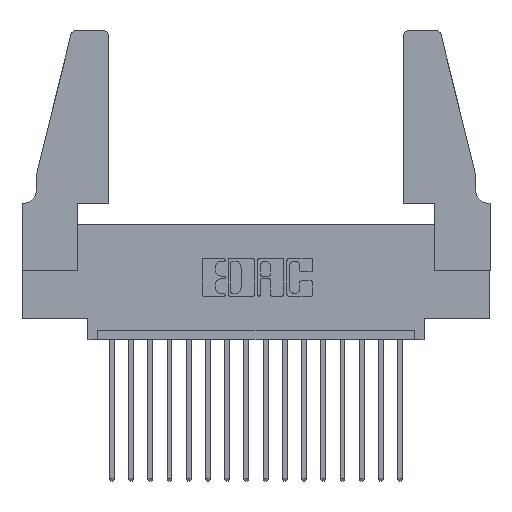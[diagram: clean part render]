
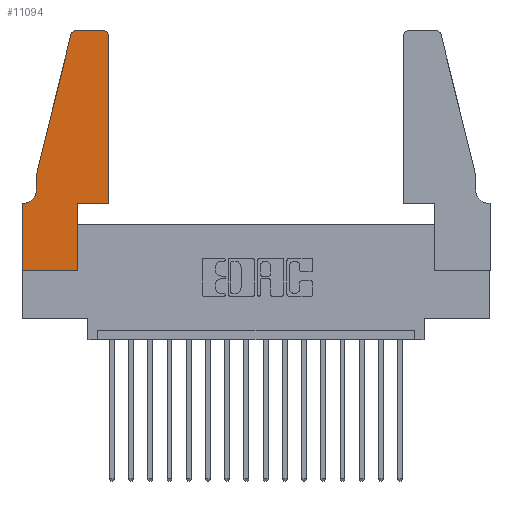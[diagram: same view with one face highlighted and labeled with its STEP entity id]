
A CAD part, top view. The second image highlights one B-rep face of the part: STEP entity #11094.
In plain terms, the highlighted planar face has unit normal (0, 0, 1).
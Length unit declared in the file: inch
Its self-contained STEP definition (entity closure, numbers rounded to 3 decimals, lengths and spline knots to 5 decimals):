
#214 = CARTESIAN_POINT ( 'NONE',  ( 0., 0., 0.37 ) ) ;
#516 = CARTESIAN_POINT ( 'NONE',  ( 0.4505, 0.35, 0.37 ) ) ;
#1029 = VECTOR ( 'NONE', #11765, 39.37008 ) ;
#1052 = EDGE_CURVE ( 'NONE', #11548, #11815, #8844, .T. ) ;
#1663 = VERTEX_POINT ( 'NONE', #3851 ) ;
#1678 = CARTESIAN_POINT ( 'NONE',  ( 0.2865, 0., 0.37 ) ) ;
#1750 = LINE ( 'NONE', #7636, #5211 ) ;
#2048 = LINE ( 'NONE', #2985, #11067 ) ;
#2205 = DIRECTION ( 'NONE',  ( 1., 0., 0. ) ) ;
#2269 = EDGE_LOOP ( 'NONE', ( #16518, #8946, #4873, #13124, #3448, #4816, #2460, #8120, #2951, #8893, #3807, #16156 ) ) ;
#2369 = DIRECTION ( 'NONE',  ( 0., 0., 1. ) ) ;
#2460 = ORIENTED_EDGE ( 'NONE', *, *, #16894, .T. ) ;
#2951 = ORIENTED_EDGE ( 'NONE', *, *, #15072, .T. ) ;
#2985 = CARTESIAN_POINT ( 'NONE',  ( 0.0755, 0.35, 0.37 ) ) ;
#3305 = VERTEX_POINT ( 'NONE', #4848 ) ;
#3448 = ORIENTED_EDGE ( 'NONE', *, *, #11821, .T. ) ;
#3489 = DIRECTION ( 'NONE',  ( 0., 1., 0. ) ) ;
#3698 = CARTESIAN_POINT ( 'NONE',  ( 0., 0.35, 0.37 ) ) ;
#3749 = VECTOR ( 'NONE', #5979, 39.37008 ) ;
#3807 = ORIENTED_EDGE ( 'NONE', *, *, #10833, .T. ) ;
#3851 = CARTESIAN_POINT ( 'NONE',  ( 0.284, 1.25, 0.37 ) ) ;
#4816 = ORIENTED_EDGE ( 'NONE', *, *, #7312, .T. ) ;
#4840 = CARTESIAN_POINT ( 'NONE',  ( 0., 0., 0.37 ) ) ;
#4848 = CARTESIAN_POINT ( 'NONE',  ( 0.0055, 0.35, 0.37 ) ) ;
#4873 = ORIENTED_EDGE ( 'NONE', *, *, #17063, .T. ) ;
#4964 = VERTEX_POINT ( 'NONE', #4840 ) ;
#4983 = EDGE_CURVE ( 'NONE', #17170, #1663, #16976, .T. ) ;
#5161 = DIRECTION ( 'NONE',  ( 1., 0., 0. ) ) ;
#5211 = VECTOR ( 'NONE', #3489, 39.37008 ) ;
#5729 = AXIS2_PLACEMENT_3D ( 'NONE', #15974, #15744, #11642 ) ;
#5944 = CARTESIAN_POINT ( 'NONE',  ( 0.2865, 0.35, 0.37 ) ) ;
#5979 = DIRECTION ( 'NONE',  ( 0., -1., 0. ) ) ;
#6034 = CARTESIAN_POINT ( 'NONE',  ( 0.4505, 0.35, 0.37 ) ) ;
#6447 = CARTESIAN_POINT ( 'NONE',  ( 0.0055, 0.42, 0.37 ) ) ;
#6463 = DIRECTION ( 'NONE',  ( -1., 0., 0. ) ) ;
#6544 = DIRECTION ( 'NONE',  ( 1., 0., 0. ) ) ;
#6773 = LINE ( 'NONE', #214, #3749 ) ;
#6805 = AXIS2_PLACEMENT_3D ( 'NONE', #12124, #14798, #6544 ) ;
#7031 = CIRCLE ( 'NONE', #11001, 0.07 ) ;
#7102 = CARTESIAN_POINT ( 'NONE',  ( 0., 0.35, 0.37 ) ) ;
#7312 = EDGE_CURVE ( 'NONE', #3305, #14896, #2048, .T. ) ;
#7475 = VECTOR ( 'NONE', #2205, 39.37008 ) ;
#7476 = VERTEX_POINT ( 'NONE', #6034 ) ;
#7528 = CARTESIAN_POINT ( 'NONE',  ( 0.0755, 0.5, 0.37 ) ) ;
#7577 = CARTESIAN_POINT ( 'NONE',  ( 0.0755, 0.5, 0.37 ) ) ;
#7585 = CARTESIAN_POINT ( 'NONE',  ( 0.2605, 1.25, 0.37 ) ) ;
#7636 = CARTESIAN_POINT ( 'NONE',  ( 0.2865, 0.35, 0.37 ) ) ;
#7899 = VECTOR ( 'NONE', #17232, 39.37008 ) ;
#8120 = ORIENTED_EDGE ( 'NONE', *, *, #15819, .T. ) ;
#8230 = AXIS2_PLACEMENT_3D ( 'NONE', #3698, #2369, #5161 ) ;
#8292 = CIRCLE ( 'NONE', #6805, 0.03 ) ;
#8754 = LINE ( 'NONE', #9001, #7475 ) ;
#8817 = DIRECTION ( 'NONE',  ( 1., 0., 0. ) ) ;
#8844 = LINE ( 'NONE', #7528, #13807 ) ;
#8893 = ORIENTED_EDGE ( 'NONE', *, *, #17524, .T. ) ;
#8946 = ORIENTED_EDGE ( 'NONE', *, *, #11992, .T. ) ;
#9001 = CARTESIAN_POINT ( 'NONE',  ( 0., 0., 0.37 ) ) ;
#9907 = VERTEX_POINT ( 'NONE', #5944 ) ;
#10202 = VECTOR ( 'NONE', #8817, 39.37008 ) ;
#10833 = EDGE_CURVE ( 'NONE', #7476, #11523, #12900, .T. ) ;
#11001 = AXIS2_PLACEMENT_3D ( 'NONE', #6447, #14585, #13121 ) ;
#11067 = VECTOR ( 'NONE', #6463, 39.37008 ) ;
#11094 = ADVANCED_FACE ( 'NONE', ( #14184 ), #13445, .T. ) ;
#11523 = VERTEX_POINT ( 'NONE', #12612 ) ;
#11548 = VERTEX_POINT ( 'NONE', #16906 ) ;
#11642 = DIRECTION ( 'NONE',  ( 1., 0., 0. ) ) ;
#11730 = CARTESIAN_POINT ( 'NONE',  ( 0.4205, 1.25, 0.37 ) ) ;
#11765 = DIRECTION ( 'NONE',  ( 0., 1., 0. ) ) ;
#11815 = VERTEX_POINT ( 'NONE', #15884 ) ;
#11821 = EDGE_CURVE ( 'NONE', #11815, #3305, #7031, .T. ) ;
#11840 = CARTESIAN_POINT ( 'NONE',  ( 0.25487, 1.22718, 0.37 ) ) ;
#11992 = EDGE_CURVE ( 'NONE', #1663, #15825, #13475, .T. ) ;
#12124 = CARTESIAN_POINT ( 'NONE',  ( 0.4205, 1.22, 0.37 ) ) ;
#12334 = VERTEX_POINT ( 'NONE', #1678 ) ;
#12612 = CARTESIAN_POINT ( 'NONE',  ( 0.4505, 1.22, 0.37 ) ) ;
#12883 = DIRECTION ( 'NONE',  ( -0.239, -0.971, 0. ) ) ;
#12900 = LINE ( 'NONE', #14616, #1029 ) ;
#13073 = DIRECTION ( 'NONE',  ( 0., -1., 0. ) ) ;
#13121 = DIRECTION ( 'NONE',  ( -1., 0., 0. ) ) ;
#13124 = ORIENTED_EDGE ( 'NONE', *, *, #1052, .T. ) ;
#13445 = PLANE ( 'NONE',  #8230 ) ;
#13475 = CIRCLE ( 'NONE', #5729, 0.03 ) ;
#13627 = LINE ( 'NONE', #516, #10202 ) ;
#13807 = VECTOR ( 'NONE', #13073, 39.37008 ) ;
#14184 = FACE_OUTER_BOUND ( 'NONE', #2269, .T. ) ;
#14585 = DIRECTION ( 'NONE',  ( 0., 0., -1. ) ) ;
#14616 = CARTESIAN_POINT ( 'NONE',  ( 0.4505, 0.35, 0.37 ) ) ;
#14798 = DIRECTION ( 'NONE',  ( 0., 0., 1. ) ) ;
#14896 = VERTEX_POINT ( 'NONE', #7102 ) ;
#15072 = EDGE_CURVE ( 'NONE', #12334, #9907, #1750, .T. ) ;
#15744 = DIRECTION ( 'NONE',  ( 0., 0., 1. ) ) ;
#15819 = EDGE_CURVE ( 'NONE', #4964, #12334, #8754, .T. ) ;
#15825 = VERTEX_POINT ( 'NONE', #11840 ) ;
#15884 = CARTESIAN_POINT ( 'NONE',  ( 0.0755, 0.42, 0.37 ) ) ;
#15974 = CARTESIAN_POINT ( 'NONE',  ( 0.284, 1.22, 0.37 ) ) ;
#15981 = EDGE_CURVE ( 'NONE', #11523, #17170, #8292, .T. ) ;
#16043 = LINE ( 'NONE', #7577, #16689 ) ;
#16156 = ORIENTED_EDGE ( 'NONE', *, *, #15981, .T. ) ;
#16518 = ORIENTED_EDGE ( 'NONE', *, *, #4983, .T. ) ;
#16689 = VECTOR ( 'NONE', #12883, 39.37008 ) ;
#16894 = EDGE_CURVE ( 'NONE', #14896, #4964, #6773, .T. ) ;
#16906 = CARTESIAN_POINT ( 'NONE',  ( 0.0755, 0.5, 0.37 ) ) ;
#16976 = LINE ( 'NONE', #7585, #7899 ) ;
#17063 = EDGE_CURVE ( 'NONE', #15825, #11548, #16043, .T. ) ;
#17170 = VERTEX_POINT ( 'NONE', #11730 ) ;
#17232 = DIRECTION ( 'NONE',  ( -1., 0., 0. ) ) ;
#17524 = EDGE_CURVE ( 'NONE', #9907, #7476, #13627, .T. ) ;
